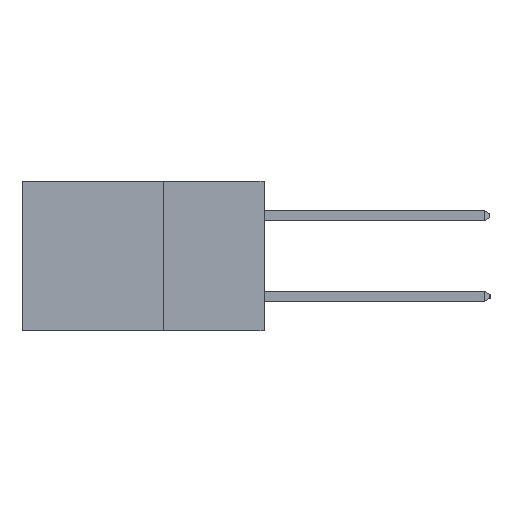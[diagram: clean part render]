
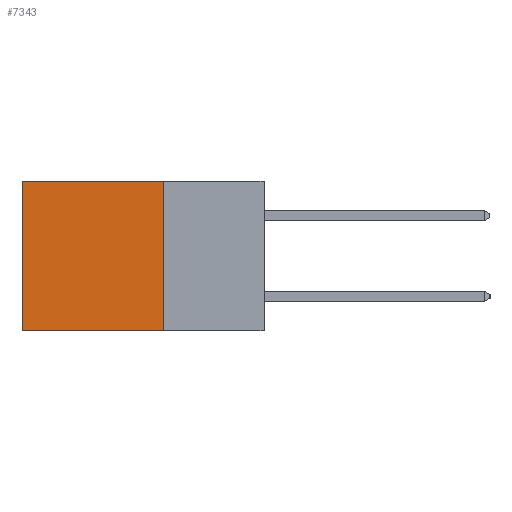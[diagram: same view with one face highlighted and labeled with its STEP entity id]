
A CAD part, left-side view. The second image highlights one B-rep face of the part: STEP entity #7343.
In plain terms, the highlighted planar face has unit normal (-1, 0, 0).
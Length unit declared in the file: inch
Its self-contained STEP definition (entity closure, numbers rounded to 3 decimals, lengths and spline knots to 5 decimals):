
#73 = ORIENTED_EDGE ( 'NONE', *, *, #10354, .F. ) ;
#277 = ORIENTED_EDGE ( 'NONE', *, *, #5650, .T. ) ;
#600 = EDGE_CURVE ( 'NONE', #1755, #10571, #9400, .T. ) ;
#1079 = ORIENTED_EDGE ( 'NONE', *, *, #600, .F. ) ;
#1158 = FACE_OUTER_BOUND ( 'NONE', #2744, .T. ) ;
#1588 = VECTOR ( 'NONE', #8451, 39.37008 ) ;
#1755 = VERTEX_POINT ( 'NONE', #4178 ) ;
#2087 = DIRECTION ( 'NONE',  ( 0., 0., -1. ) ) ;
#2154 = VECTOR ( 'NONE', #6852, 39.37008 ) ;
#2192 = CARTESIAN_POINT ( 'NONE',  ( 0.2615, 0.6, -0.37 ) ) ;
#2744 = EDGE_LOOP ( 'NONE', ( #4969, #73, #1079, #277 ) ) ;
#2949 = VERTEX_POINT ( 'NONE', #8437 ) ;
#3683 = VECTOR ( 'NONE', #2087, 39.37008 ) ;
#3796 = CARTESIAN_POINT ( 'NONE',  ( 0.2615, 0.25, -0.37 ) ) ;
#3975 = LINE ( 'NONE', #2192, #3683 ) ;
#4178 = CARTESIAN_POINT ( 'NONE',  ( 0.2615, 0.25, 0. ) ) ;
#4383 = AXIS2_PLACEMENT_3D ( 'NONE', #6649, #6394, #6379 ) ;
#4969 = ORIENTED_EDGE ( 'NONE', *, *, #7571, .T. ) ;
#5340 = LINE ( 'NONE', #6895, #7658 ) ;
#5650 = EDGE_CURVE ( 'NONE', #1755, #11850, #5340, .T. ) ;
#6379 = DIRECTION ( 'NONE',  ( 0., 0., -1. ) ) ;
#6394 = DIRECTION ( 'NONE',  ( 1., 0., 0. ) ) ;
#6447 = PLANE ( 'NONE',  #4383 ) ;
#6613 = CARTESIAN_POINT ( 'NONE',  ( 0.2615, 0.25, -0.37 ) ) ;
#6646 = CARTESIAN_POINT ( 'NONE',  ( 0.2615, 0.25, -0.37 ) ) ;
#6649 = CARTESIAN_POINT ( 'NONE',  ( 0.2615, 0.25, -0.37 ) ) ;
#6766 = DIRECTION ( 'NONE',  ( 0., 1., 0. ) ) ;
#6852 = DIRECTION ( 'NONE',  ( 0., 1., 0. ) ) ;
#6895 = CARTESIAN_POINT ( 'NONE',  ( 0.2615, 0.25, 0. ) ) ;
#7343 = ADVANCED_FACE ( 'NONE', ( #1158 ), #6447, .F. ) ;
#7380 = LINE ( 'NONE', #6646, #2154 ) ;
#7571 = EDGE_CURVE ( 'NONE', #11850, #2949, #3975, .T. ) ;
#7658 = VECTOR ( 'NONE', #6766, 39.37008 ) ;
#8437 = CARTESIAN_POINT ( 'NONE',  ( 0.2615, 0.6, -0.37 ) ) ;
#8451 = DIRECTION ( 'NONE',  ( 0., 0., -1. ) ) ;
#9369 = CARTESIAN_POINT ( 'NONE',  ( 0.2615, 0.6, 0. ) ) ;
#9400 = LINE ( 'NONE', #6613, #1588 ) ;
#10354 = EDGE_CURVE ( 'NONE', #10571, #2949, #7380, .T. ) ;
#10571 = VERTEX_POINT ( 'NONE', #3796 ) ;
#11850 = VERTEX_POINT ( 'NONE', #9369 ) ;
